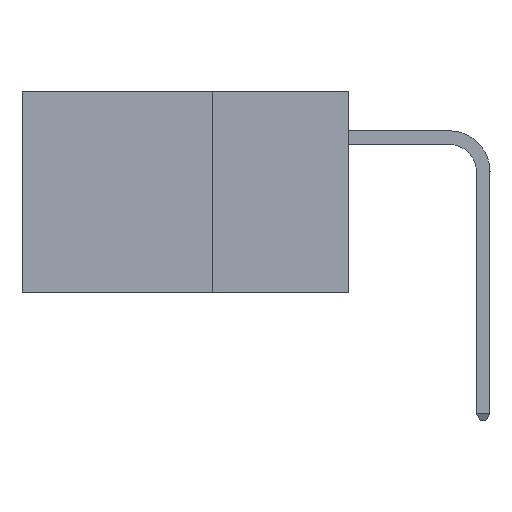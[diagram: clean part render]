
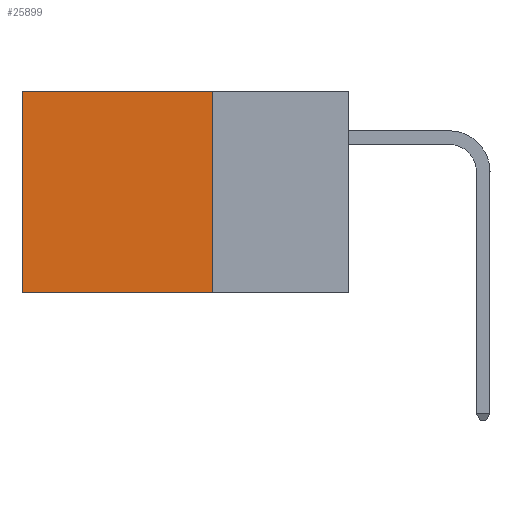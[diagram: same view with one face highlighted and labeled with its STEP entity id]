
A CAD part, left-side view. The second image highlights one B-rep face of the part: STEP entity #25899.
In plain terms, the highlighted planar face has unit normal (-1, 0, 0).
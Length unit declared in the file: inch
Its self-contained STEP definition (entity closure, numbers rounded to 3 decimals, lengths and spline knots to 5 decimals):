
#588 = VECTOR ( 'NONE', #22264, 39.37008 ) ;
#1699 = EDGE_CURVE ( 'NONE', #40254, #13746, #35392, .T. ) ;
#1878 = CARTESIAN_POINT ( 'NONE',  ( 0.2875, 0.25, -0.37 ) ) ;
#3260 = CARTESIAN_POINT ( 'NONE',  ( 0.2875, 0.6, 0. ) ) ;
#3725 = EDGE_CURVE ( 'NONE', #37906, #13746, #13811, .T. ) ;
#3746 = VERTEX_POINT ( 'NONE', #29437 ) ;
#4692 = VECTOR ( 'NONE', #19082, 39.37008 ) ;
#8486 = ORIENTED_EDGE ( 'NONE', *, *, #3725, .T. ) ;
#10253 = CARTESIAN_POINT ( 'NONE',  ( 0.2875, 0.6, 0. ) ) ;
#12128 = ORIENTED_EDGE ( 'NONE', *, *, #1699, .F. ) ;
#13626 = CARTESIAN_POINT ( 'NONE',  ( 0.2875, 0.6, -0.37 ) ) ;
#13746 = VERTEX_POINT ( 'NONE', #13626 ) ;
#13811 = LINE ( 'NONE', #10253, #588 ) ;
#14789 = ORIENTED_EDGE ( 'NONE', *, *, #39244, .T. ) ;
#14833 = EDGE_LOOP ( 'NONE', ( #8486, #12128, #26676, #14789 ) ) ;
#15610 = FACE_OUTER_BOUND ( 'NONE', #14833, .T. ) ;
#15666 = DIRECTION ( 'NONE',  ( 1., 0., 0. ) ) ;
#15799 = CARTESIAN_POINT ( 'NONE',  ( 0.2875, 0.25, 0. ) ) ;
#19082 = DIRECTION ( 'NONE',  ( 0., 1., 0. ) ) ;
#21101 = AXIS2_PLACEMENT_3D ( 'NONE', #15799, #15666, #40246 ) ;
#21157 = DIRECTION ( 'NONE',  ( 0., 0., -1. ) ) ;
#22264 = DIRECTION ( 'NONE',  ( 0., 0., -1. ) ) ;
#22579 = DIRECTION ( 'NONE',  ( 0., 1., 0. ) ) ;
#24136 = CARTESIAN_POINT ( 'NONE',  ( 0.2875, 0.25, -0.37 ) ) ;
#25456 = VECTOR ( 'NONE', #21157, 39.37008 ) ;
#25835 = CARTESIAN_POINT ( 'NONE',  ( 0.2875, 0.25, 0. ) ) ;
#25899 = ADVANCED_FACE ( 'NONE', ( #15610 ), #37012, .F. ) ;
#26676 = ORIENTED_EDGE ( 'NONE', *, *, #38363, .F. ) ;
#29437 = CARTESIAN_POINT ( 'NONE',  ( 0.2875, 0.25, 0. ) ) ;
#32241 = LINE ( 'NONE', #40154, #25456 ) ;
#35392 = LINE ( 'NONE', #1878, #4692 ) ;
#35647 = VECTOR ( 'NONE', #22579, 39.37008 ) ;
#37012 = PLANE ( 'NONE',  #21101 ) ;
#37040 = LINE ( 'NONE', #25835, #35647 ) ;
#37906 = VERTEX_POINT ( 'NONE', #3260 ) ;
#38363 = EDGE_CURVE ( 'NONE', #3746, #40254, #32241, .T. ) ;
#39244 = EDGE_CURVE ( 'NONE', #3746, #37906, #37040, .T. ) ;
#40154 = CARTESIAN_POINT ( 'NONE',  ( 0.2875, 0.25, 0. ) ) ;
#40246 = DIRECTION ( 'NONE',  ( 0., 0., -1. ) ) ;
#40254 = VERTEX_POINT ( 'NONE', #24136 ) ;
